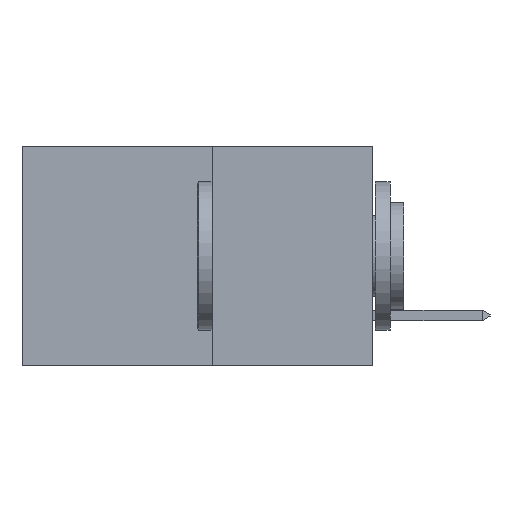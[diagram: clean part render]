
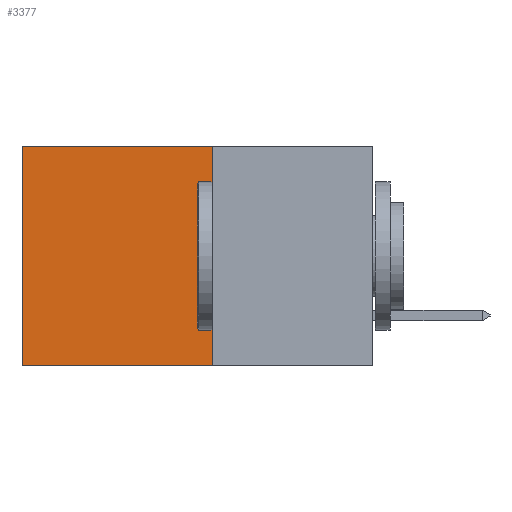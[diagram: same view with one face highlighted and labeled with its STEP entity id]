
A CAD part, left-side view. The second image highlights one B-rep face of the part: STEP entity #3377.
In plain terms, the highlighted planar face has unit normal (-1, 0, 0).
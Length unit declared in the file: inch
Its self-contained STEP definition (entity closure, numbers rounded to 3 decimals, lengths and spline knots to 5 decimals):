
#1230 = VECTOR ( 'NONE', #8447, 39.37008 ) ;
#1305 = FACE_OUTER_BOUND ( 'NONE', #21547, .T. ) ;
#1792 = LINE ( 'NONE', #6778, #1230 ) ;
#1968 = DIRECTION ( 'NONE',  ( 1., 0., 0. ) ) ;
#2098 = DIRECTION ( 'NONE',  ( 0., 1., 0. ) ) ;
#3213 = CARTESIAN_POINT ( 'NONE',  ( 0.277, 0.59, -0.37 ) ) ;
#3377 = ADVANCED_FACE ( 'NONE', ( #1305 ), #11887, .F. ) ;
#5341 = VERTEX_POINT ( 'NONE', #3213 ) ;
#5539 = LINE ( 'NONE', #16107, #9447 ) ;
#6778 = CARTESIAN_POINT ( 'NONE',  ( 0.277, 0.27, -0.37 ) ) ;
#7020 = CARTESIAN_POINT ( 'NONE',  ( 0.277, 0.27, -0.37 ) ) ;
#7121 = EDGE_CURVE ( 'NONE', #16245, #12136, #1792, .T. ) ;
#7593 = DIRECTION ( 'NONE',  ( 0., 0., -1. ) ) ;
#8266 = EDGE_CURVE ( 'NONE', #12136, #5341, #9381, .T. ) ;
#8334 = ORIENTED_EDGE ( 'NONE', *, *, #19366, .T. ) ;
#8447 = DIRECTION ( 'NONE',  ( 0., 0., -1. ) ) ;
#9381 = LINE ( 'NONE', #13086, #17896 ) ;
#9447 = VECTOR ( 'NONE', #7593, 39.37008 ) ;
#10475 = CARTESIAN_POINT ( 'NONE',  ( 0.277, 0.27, 0. ) ) ;
#11806 = CARTESIAN_POINT ( 'NONE',  ( 0.277, 0.27, -0.37 ) ) ;
#11887 = PLANE ( 'NONE',  #17304 ) ;
#12136 = VERTEX_POINT ( 'NONE', #11806 ) ;
#12239 = ORIENTED_EDGE ( 'NONE', *, *, #18483, .T. ) ;
#12319 = VECTOR ( 'NONE', #2098, 39.37008 ) ;
#13086 = CARTESIAN_POINT ( 'NONE',  ( 0.277, 0.27, -0.37 ) ) ;
#14826 = DIRECTION ( 'NONE',  ( 0., 1., 0. ) ) ;
#15681 = CARTESIAN_POINT ( 'NONE',  ( 0.277, 0.27, 0. ) ) ;
#16107 = CARTESIAN_POINT ( 'NONE',  ( 0.277, 0.59, -0.37 ) ) ;
#16245 = VERTEX_POINT ( 'NONE', #15681 ) ;
#16718 = ORIENTED_EDGE ( 'NONE', *, *, #7121, .F. ) ;
#17238 = DIRECTION ( 'NONE',  ( 0., 0., -1. ) ) ;
#17304 = AXIS2_PLACEMENT_3D ( 'NONE', #7020, #1968, #17238 ) ;
#17896 = VECTOR ( 'NONE', #14826, 39.37008 ) ;
#18483 = EDGE_CURVE ( 'NONE', #21945, #5341, #5539, .T. ) ;
#19363 = ORIENTED_EDGE ( 'NONE', *, *, #8266, .F. ) ;
#19366 = EDGE_CURVE ( 'NONE', #16245, #21945, #21853, .T. ) ;
#21147 = CARTESIAN_POINT ( 'NONE',  ( 0.277, 0.59, 0. ) ) ;
#21547 = EDGE_LOOP ( 'NONE', ( #12239, #19363, #16718, #8334 ) ) ;
#21853 = LINE ( 'NONE', #10475, #12319 ) ;
#21945 = VERTEX_POINT ( 'NONE', #21147 ) ;
